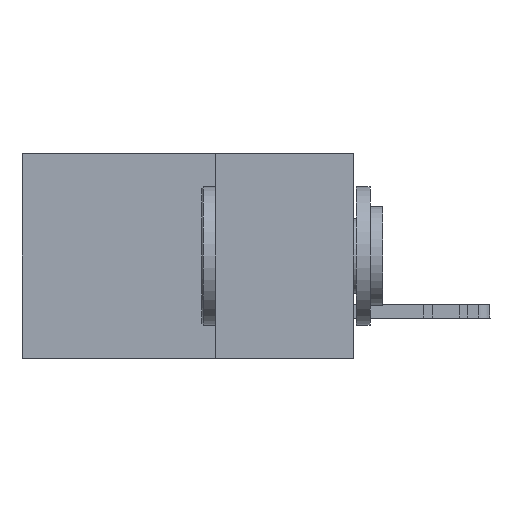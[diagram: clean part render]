
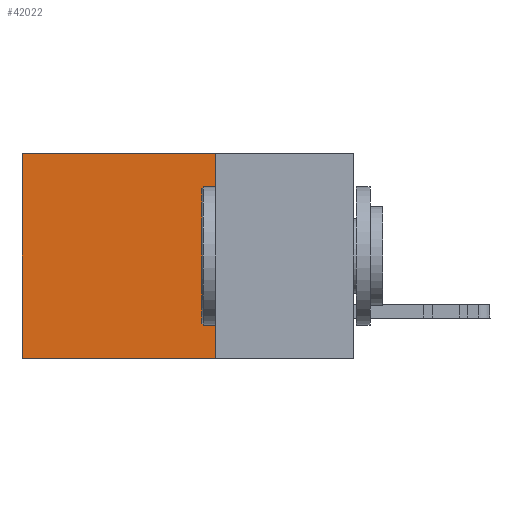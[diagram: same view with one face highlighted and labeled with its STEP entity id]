
A CAD part, left-side view. The second image highlights one B-rep face of the part: STEP entity #42022.
In plain terms, the highlighted planar face has unit normal (-1, 0, 0).
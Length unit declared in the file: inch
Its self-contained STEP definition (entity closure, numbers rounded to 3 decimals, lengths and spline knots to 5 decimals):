
#1867 = EDGE_CURVE ( 'NONE', #8892, #41735, #21116, .T. ) ;
#2461 = EDGE_LOOP ( 'NONE', ( #17486, #5749, #10202, #44070 ) ) ;
#3278 = VECTOR ( 'NONE', #15724, 39.37008 ) ;
#5718 = VERTEX_POINT ( 'NONE', #48935 ) ;
#5749 = ORIENTED_EDGE ( 'NONE', *, *, #25496, .F. ) ;
#7296 = DIRECTION ( 'NONE',  ( 0., 0., -1. ) ) ;
#8892 = VERTEX_POINT ( 'NONE', #28800 ) ;
#8920 = CARTESIAN_POINT ( 'NONE',  ( 0.2875, 0.25, -0.37 ) ) ;
#9350 = LINE ( 'NONE', #8920, #11912 ) ;
#10202 = ORIENTED_EDGE ( 'NONE', *, *, #15228, .F. ) ;
#10957 = PLANE ( 'NONE',  #48177 ) ;
#11912 = VECTOR ( 'NONE', #46202, 39.37008 ) ;
#15228 = EDGE_CURVE ( 'NONE', #8892, #47019, #44575, .T. ) ;
#15724 = DIRECTION ( 'NONE',  ( 0., 0., -1. ) ) ;
#17486 = ORIENTED_EDGE ( 'NONE', *, *, #47136, .T. ) ;
#18804 = DIRECTION ( 'NONE',  ( 1., 0., 0. ) ) ;
#20247 = CARTESIAN_POINT ( 'NONE',  ( 0.2875, 0.6, 0. ) ) ;
#21116 = LINE ( 'NONE', #45925, #48064 ) ;
#21562 = LINE ( 'NONE', #35742, #3278 ) ;
#25496 = EDGE_CURVE ( 'NONE', #47019, #5718, #9350, .T. ) ;
#28800 = CARTESIAN_POINT ( 'NONE',  ( 0.2875, 0.25, 0. ) ) ;
#33594 = DIRECTION ( 'NONE',  ( 0., 1., 0. ) ) ;
#34375 = DIRECTION ( 'NONE',  ( 0., 0., -1. ) ) ;
#34623 = CARTESIAN_POINT ( 'NONE',  ( 0.2875, 0.25, -0.37 ) ) ;
#35742 = CARTESIAN_POINT ( 'NONE',  ( 0.2875, 0.6, 0. ) ) ;
#41070 = FACE_OUTER_BOUND ( 'NONE', #2461, .T. ) ;
#41735 = VERTEX_POINT ( 'NONE', #20247 ) ;
#42022 = ADVANCED_FACE ( 'NONE', ( #41070 ), #10957, .F. ) ;
#44070 = ORIENTED_EDGE ( 'NONE', *, *, #1867, .T. ) ;
#44575 = LINE ( 'NONE', #50232, #47135 ) ;
#45457 = CARTESIAN_POINT ( 'NONE',  ( 0.2875, 0.25, 0. ) ) ;
#45925 = CARTESIAN_POINT ( 'NONE',  ( 0.2875, 0.25, 0. ) ) ;
#46202 = DIRECTION ( 'NONE',  ( 0., 1., 0. ) ) ;
#47019 = VERTEX_POINT ( 'NONE', #34623 ) ;
#47135 = VECTOR ( 'NONE', #7296, 39.37008 ) ;
#47136 = EDGE_CURVE ( 'NONE', #41735, #5718, #21562, .T. ) ;
#48064 = VECTOR ( 'NONE', #33594, 39.37008 ) ;
#48177 = AXIS2_PLACEMENT_3D ( 'NONE', #45457, #18804, #34375 ) ;
#48935 = CARTESIAN_POINT ( 'NONE',  ( 0.2875, 0.6, -0.37 ) ) ;
#50232 = CARTESIAN_POINT ( 'NONE',  ( 0.2875, 0.25, 0. ) ) ;
